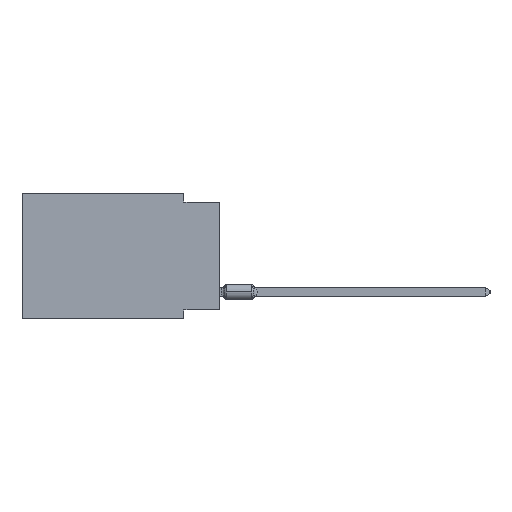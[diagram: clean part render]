
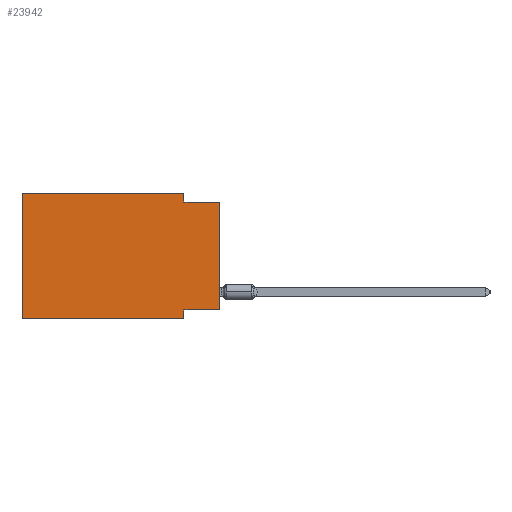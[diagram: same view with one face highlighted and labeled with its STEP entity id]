
A CAD part, left-side view. The second image highlights one B-rep face of the part: STEP entity #23942.
In plain terms, the highlighted planar face has unit normal (-1, 0, 0).
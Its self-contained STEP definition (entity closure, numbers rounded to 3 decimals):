
#266 = VECTOR ( 'NONE', #28137, 1000. ) ;
#1301 = LINE ( 'NONE', #7916, #59037 ) ;
#1313 = VERTEX_POINT ( 'NONE', #55292 ) ;
#3494 = VERTEX_POINT ( 'NONE', #62041 ) ;
#5033 = ORIENTED_EDGE ( 'NONE', *, *, #44496, .F. ) ;
#7227 = VERTEX_POINT ( 'NONE', #71318 ) ;
#7916 = CARTESIAN_POINT ( 'NONE',  ( 0., 2.54, 0. ) ) ;
#9947 = VECTOR ( 'NONE', #43122, 1000. ) ;
#10297 = LINE ( 'NONE', #45762, #68458 ) ;
#10377 = ORIENTED_EDGE ( 'NONE', *, *, #40959, .F. ) ;
#11733 = CARTESIAN_POINT ( 'NONE',  ( 0., 2.54, 0. ) ) ;
#14748 = CARTESIAN_POINT ( 'NONE',  ( 0., 0., -0.635 ) ) ;
#14814 = DIRECTION ( 'NONE',  ( 1., 0., 0. ) ) ;
#16858 = EDGE_CURVE ( 'NONE', #3494, #31877, #58769, .T. ) ;
#20195 = VECTOR ( 'NONE', #33586, 1000. ) ;
#22679 = VERTEX_POINT ( 'NONE', #45902 ) ;
#22828 = CARTESIAN_POINT ( 'NONE',  ( 0., 2.54, -8.89 ) ) ;
#22946 = DIRECTION ( 'NONE',  ( 0., 0., 1. ) ) ;
#23942 = ADVANCED_FACE ( 'NONE', ( #86703 ), #36566, .F. ) ;
#24032 = DIRECTION ( 'NONE',  ( 0., 0., 1. ) ) ;
#25777 = EDGE_CURVE ( 'NONE', #1313, #37102, #79366, .T. ) ;
#25895 = EDGE_CURVE ( 'NONE', #22679, #7227, #10297, .T. ) ;
#27589 = DIRECTION ( 'NONE',  ( 0., 0., -1. ) ) ;
#28137 = DIRECTION ( 'NONE',  ( 0., -1., 0. ) ) ;
#29235 = CARTESIAN_POINT ( 'NONE',  ( 0., 13.97, 0. ) ) ;
#29527 = ORIENTED_EDGE ( 'NONE', *, *, #48121, .F. ) ;
#30333 = CARTESIAN_POINT ( 'NONE',  ( 0., 2.54, -0.635 ) ) ;
#30569 = ORIENTED_EDGE ( 'NONE', *, *, #37594, .T. ) ;
#31877 = VERTEX_POINT ( 'NONE', #88221 ) ;
#33586 = DIRECTION ( 'NONE',  ( 0., 1., 0. ) ) ;
#36314 = ORIENTED_EDGE ( 'NONE', *, *, #25777, .F. ) ;
#36503 = LINE ( 'NONE', #14748, #9947 ) ;
#36566 = PLANE ( 'NONE',  #66699 ) ;
#37102 = VERTEX_POINT ( 'NONE', #11733 ) ;
#37260 = DIRECTION ( 'NONE',  ( 0., 0., -1. ) ) ;
#37361 = VECTOR ( 'NONE', #22946, 1000. ) ;
#37594 = EDGE_CURVE ( 'NONE', #45195, #31877, #41868, .T. ) ;
#38561 = VECTOR ( 'NONE', #51670, 1000. ) ;
#40256 = ORIENTED_EDGE ( 'NONE', *, *, #50647, .F. ) ;
#40830 = VERTEX_POINT ( 'NONE', #30333 ) ;
#40959 = EDGE_CURVE ( 'NONE', #22679, #3494, #76170, .T. ) ;
#41868 = LINE ( 'NONE', #93409, #266 ) ;
#43122 = DIRECTION ( 'NONE',  ( 0., -1., 0. ) ) ;
#43759 = CARTESIAN_POINT ( 'NONE',  ( 0., 13.97, 0. ) ) ;
#44496 = EDGE_CURVE ( 'NONE', #40830, #7227, #36503, .T. ) ;
#45195 = VERTEX_POINT ( 'NONE', #76985 ) ;
#45762 = CARTESIAN_POINT ( 'NONE',  ( 0., 0., 0. ) ) ;
#45902 = CARTESIAN_POINT ( 'NONE',  ( 0., 0., -8.255 ) ) ;
#48121 = EDGE_CURVE ( 'NONE', #45195, #1313, #79711, .T. ) ;
#50647 = EDGE_CURVE ( 'NONE', #37102, #40830, #1301, .T. ) ;
#51670 = DIRECTION ( 'NONE',  ( 0., 0., -1. ) ) ;
#55292 = CARTESIAN_POINT ( 'NONE',  ( 0., 13.97, 0. ) ) ;
#58078 = DIRECTION ( 'NONE',  ( 0., -1., 0. ) ) ;
#58769 = LINE ( 'NONE', #22828, #38561 ) ;
#59037 = VECTOR ( 'NONE', #37260, 1000. ) ;
#61965 = CARTESIAN_POINT ( 'NONE',  ( 0., 0., -8.255 ) ) ;
#62041 = CARTESIAN_POINT ( 'NONE',  ( 0., 2.54, -8.255 ) ) ;
#63903 = VECTOR ( 'NONE', #58078, 1000. ) ;
#66699 = AXIS2_PLACEMENT_3D ( 'NONE', #79138, #14814, #27589 ) ;
#68458 = VECTOR ( 'NONE', #24032, 1000. ) ;
#69872 = EDGE_LOOP ( 'NONE', ( #73133, #5033, #40256, #36314, #29527, #30569, #73112, #10377 ) ) ;
#71318 = CARTESIAN_POINT ( 'NONE',  ( 0., 0., -0.635 ) ) ;
#73112 = ORIENTED_EDGE ( 'NONE', *, *, #16858, .F. ) ;
#73133 = ORIENTED_EDGE ( 'NONE', *, *, #25895, .T. ) ;
#76170 = LINE ( 'NONE', #61965, #20195 ) ;
#76985 = CARTESIAN_POINT ( 'NONE',  ( 0., 13.97, -8.89 ) ) ;
#79138 = CARTESIAN_POINT ( 'NONE',  ( 0., 13.97, 0. ) ) ;
#79366 = LINE ( 'NONE', #29235, #63903 ) ;
#79711 = LINE ( 'NONE', #43759, #37361 ) ;
#86703 = FACE_OUTER_BOUND ( 'NONE', #69872, .T. ) ;
#88221 = CARTESIAN_POINT ( 'NONE',  ( 0., 2.54, -8.89 ) ) ;
#93409 = CARTESIAN_POINT ( 'NONE',  ( 0., 13.97, -8.89 ) ) ;
